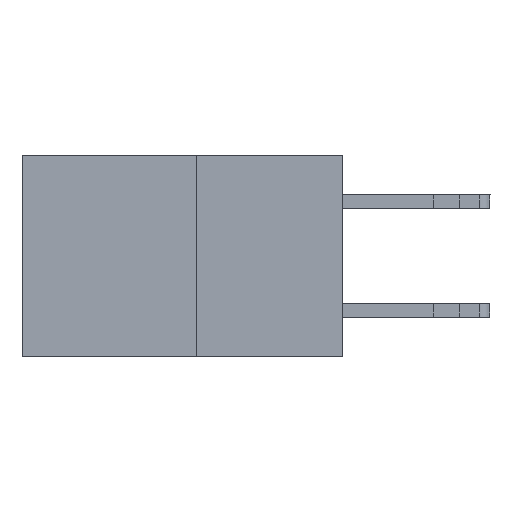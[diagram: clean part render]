
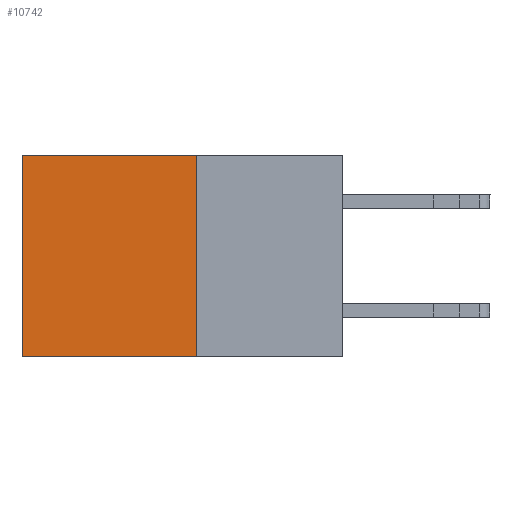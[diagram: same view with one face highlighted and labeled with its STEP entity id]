
A CAD part, left-side view. The second image highlights one B-rep face of the part: STEP entity #10742.
In plain terms, the highlighted planar face has unit normal (-1, 0, 0).
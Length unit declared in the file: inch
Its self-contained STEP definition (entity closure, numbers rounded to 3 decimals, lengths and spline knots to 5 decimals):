
#204 = VERTEX_POINT ( 'NONE', #15881 ) ;
#3248 = VERTEX_POINT ( 'NONE', #25333 ) ;
#4366 = ORIENTED_EDGE ( 'NONE', *, *, #22139, .T. ) ;
#5378 = EDGE_CURVE ( 'NONE', #3248, #21464, #23328, .T. ) ;
#5441 = CARTESIAN_POINT ( 'NONE',  ( 0.277, 0.27, -0.37 ) ) ;
#5886 = CARTESIAN_POINT ( 'NONE',  ( 0.277, 0.27, -0.37 ) ) ;
#8369 = LINE ( 'NONE', #17143, #14955 ) ;
#9224 = CARTESIAN_POINT ( 'NONE',  ( 0.277, 0.27, -0.37 ) ) ;
#9370 = VECTOR ( 'NONE', #27449, 39.37008 ) ;
#9929 = AXIS2_PLACEMENT_3D ( 'NONE', #5886, #12408, #23177 ) ;
#10035 = CARTESIAN_POINT ( 'NONE',  ( 0.277, 0.27, -0.37 ) ) ;
#10373 = ORIENTED_EDGE ( 'NONE', *, *, #16005, .T. ) ;
#10742 = ADVANCED_FACE ( 'NONE', ( #23308 ), #11996, .F. ) ;
#11996 = PLANE ( 'NONE',  #9929 ) ;
#12408 = DIRECTION ( 'NONE',  ( 1., 0., 0. ) ) ;
#14955 = VECTOR ( 'NONE', #27373, 39.37008 ) ;
#15197 = DIRECTION ( 'NONE',  ( 0., 1., 0. ) ) ;
#15208 = EDGE_CURVE ( 'NONE', #21464, #204, #26637, .T. ) ;
#15814 = ORIENTED_EDGE ( 'NONE', *, *, #15208, .F. ) ;
#15881 = CARTESIAN_POINT ( 'NONE',  ( 0.277, 0.59, -0.37 ) ) ;
#16005 = EDGE_CURVE ( 'NONE', #3248, #26303, #26101, .T. ) ;
#17143 = CARTESIAN_POINT ( 'NONE',  ( 0.277, 0.59, -0.37 ) ) ;
#17259 = VECTOR ( 'NONE', #15197, 39.37008 ) ;
#19007 = CARTESIAN_POINT ( 'NONE',  ( 0.277, 0.59, 0. ) ) ;
#19178 = CARTESIAN_POINT ( 'NONE',  ( 0.277, 0.27, 0. ) ) ;
#21464 = VERTEX_POINT ( 'NONE', #5441 ) ;
#21652 = EDGE_LOOP ( 'NONE', ( #4366, #15814, #25292, #10373 ) ) ;
#22139 = EDGE_CURVE ( 'NONE', #26303, #204, #8369, .T. ) ;
#23177 = DIRECTION ( 'NONE',  ( 0., 0., -1. ) ) ;
#23308 = FACE_OUTER_BOUND ( 'NONE', #21652, .T. ) ;
#23328 = LINE ( 'NONE', #10035, #9370 ) ;
#24227 = DIRECTION ( 'NONE',  ( 0., 1., 0. ) ) ;
#25292 = ORIENTED_EDGE ( 'NONE', *, *, #5378, .F. ) ;
#25333 = CARTESIAN_POINT ( 'NONE',  ( 0.277, 0.27, 0. ) ) ;
#26101 = LINE ( 'NONE', #19178, #17259 ) ;
#26303 = VERTEX_POINT ( 'NONE', #19007 ) ;
#26637 = LINE ( 'NONE', #9224, #26748 ) ;
#26748 = VECTOR ( 'NONE', #24227, 39.37008 ) ;
#27373 = DIRECTION ( 'NONE',  ( 0., 0., -1. ) ) ;
#27449 = DIRECTION ( 'NONE',  ( 0., 0., -1. ) ) ;
